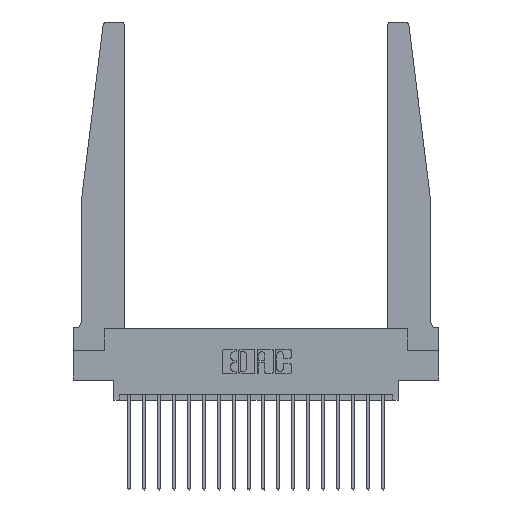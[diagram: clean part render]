
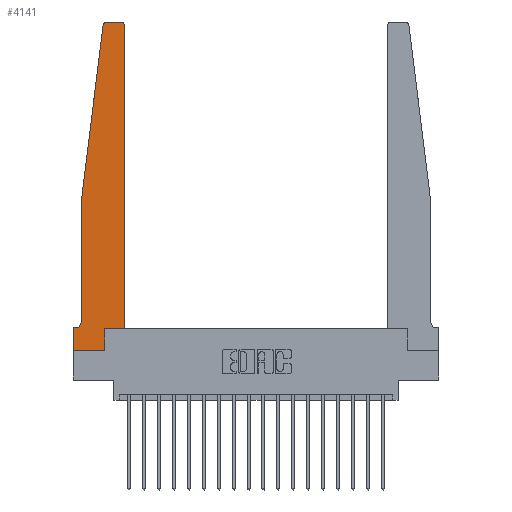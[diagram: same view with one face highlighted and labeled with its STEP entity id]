
A CAD part, top view. The second image highlights one B-rep face of the part: STEP entity #4141.
In plain terms, the highlighted planar face has unit normal (0, 0, 1).
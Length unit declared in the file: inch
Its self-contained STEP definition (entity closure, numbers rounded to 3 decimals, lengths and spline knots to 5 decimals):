
#254 = VERTEX_POINT ( 'NONE', #12240 ) ;
#516 = CARTESIAN_POINT ( 'NONE',  ( 0., 0., 0.37 ) ) ;
#524 = ORIENTED_EDGE ( 'NONE', *, *, #786, .T. ) ;
#786 = EDGE_CURVE ( 'NONE', #16595, #11961, #11822, .T. ) ;
#792 = VERTEX_POINT ( 'NONE', #1582 ) ;
#1427 = EDGE_CURVE ( 'NONE', #10707, #254, #6270, .T. ) ;
#1582 = CARTESIAN_POINT ( 'NONE',  ( 0., 0.1875, 0.37 ) ) ;
#1601 = DIRECTION ( 'NONE',  ( -0.122, -0.992, 0. ) ) ;
#1980 = ORIENTED_EDGE ( 'NONE', *, *, #9373, .T. ) ;
#2039 = CARTESIAN_POINT ( 'NONE',  ( 0., 0., 0.37 ) ) ;
#2236 = ORIENTED_EDGE ( 'NONE', *, *, #12065, .T. ) ;
#2300 = CARTESIAN_POINT ( 'NONE',  ( 0.065, 0.1875, 0.37 ) ) ;
#2331 = EDGE_LOOP ( 'NONE', ( #16674, #18493, #1980, #10214, #2236, #14334, #15579, #4472, #19203, #524, #14915, #15551 ) ) ;
#2355 = FACE_OUTER_BOUND ( 'NONE', #2331, .T. ) ;
#3036 = VERTEX_POINT ( 'NONE', #16102 ) ;
#3189 = VECTOR ( 'NONE', #12989, 39.37008 ) ;
#3217 = LINE ( 'NONE', #516, #19069 ) ;
#3950 = DIRECTION ( 'NONE',  ( -1., 0., 0. ) ) ;
#4141 = ADVANCED_FACE ( 'NONE', ( #2355 ), #6121, .T. ) ;
#4194 = EDGE_CURVE ( 'NONE', #8785, #9283, #17755, .T. ) ;
#4259 = CARTESIAN_POINT ( 'NONE',  ( 0.2605, 0.18, 0.37 ) ) ;
#4472 = ORIENTED_EDGE ( 'NONE', *, *, #1427, .T. ) ;
#4792 = AXIS2_PLACEMENT_3D ( 'NONE', #16905, #7654, #18449 ) ;
#4991 = DIRECTION ( 'NONE',  ( 0., 0., 1. ) ) ;
#5157 = DIRECTION ( 'NONE',  ( 0., 0., -1. ) ) ;
#5566 = CARTESIAN_POINT ( 'NONE',  ( 0.27653, 2.72, 0.37 ) ) ;
#5692 = LINE ( 'NONE', #12302, #8798 ) ;
#6121 = PLANE ( 'NONE',  #4792 ) ;
#6270 = LINE ( 'NONE', #7575, #18107 ) ;
#6414 = DIRECTION ( 'NONE',  ( 0., 1., 0. ) ) ;
#7090 = DIRECTION ( 'NONE',  ( 1., 0., 0. ) ) ;
#7575 = CARTESIAN_POINT ( 'NONE',  ( 0., 0., 0.37 ) ) ;
#7654 = DIRECTION ( 'NONE',  ( 0., 0., 1. ) ) ;
#7961 = CARTESIAN_POINT ( 'NONE',  ( 0.425, 0.18, 0.37 ) ) ;
#8785 = VERTEX_POINT ( 'NONE', #10706 ) ;
#8798 = VECTOR ( 'NONE', #1601, 39.37008 ) ;
#8868 = LINE ( 'NONE', #14680, #17066 ) ;
#9215 = EDGE_CURVE ( 'NONE', #13686, #16363, #15149, .T. ) ;
#9283 = VERTEX_POINT ( 'NONE', #19532 ) ;
#9373 = EDGE_CURVE ( 'NONE', #16363, #8785, #5692, .T. ) ;
#10214 = ORIENTED_EDGE ( 'NONE', *, *, #4194, .T. ) ;
#10706 = CARTESIAN_POINT ( 'NONE',  ( 0.065, 1.25, 0.37 ) ) ;
#10707 = VERTEX_POINT ( 'NONE', #2039 ) ;
#10833 = LINE ( 'NONE', #2300, #3189 ) ;
#11227 = EDGE_CURVE ( 'NONE', #11961, #13892, #16921, .T. ) ;
#11345 = EDGE_CURVE ( 'NONE', #792, #10707, #3217, .T. ) ;
#11695 = CARTESIAN_POINT ( 'NONE',  ( 0.27653, 2.75, 0.37 ) ) ;
#11822 = LINE ( 'NONE', #12413, #14980 ) ;
#11961 = VERTEX_POINT ( 'NONE', #15616 ) ;
#12065 = EDGE_CURVE ( 'NONE', #9283, #3036, #15671, .T. ) ;
#12240 = CARTESIAN_POINT ( 'NONE',  ( 0.2605, 0., 0.37 ) ) ;
#12302 = CARTESIAN_POINT ( 'NONE',  ( 0.065, 1.25, 0.37 ) ) ;
#12355 = AXIS2_PLACEMENT_3D ( 'NONE', #5566, #16315, #7090 ) ;
#12378 = AXIS2_PLACEMENT_3D ( 'NONE', #14344, #5157, #15896 ) ;
#12391 = CARTESIAN_POINT ( 'NONE',  ( 0.065, 1.25, 0.37 ) ) ;
#12413 = CARTESIAN_POINT ( 'NONE',  ( 0.425, 0.18, 0.37 ) ) ;
#12776 = VECTOR ( 'NONE', #6414, 39.37008 ) ;
#12989 = DIRECTION ( 'NONE',  ( -1., 0., 0. ) ) ;
#13686 = VERTEX_POINT ( 'NONE', #11695 ) ;
#13892 = VERTEX_POINT ( 'NONE', #15277 ) ;
#14163 = CARTESIAN_POINT ( 'NONE',  ( 0.395, 2.72, 0.37 ) ) ;
#14173 = VECTOR ( 'NONE', #18573, 39.37008 ) ;
#14334 = ORIENTED_EDGE ( 'NONE', *, *, #18306, .T. ) ;
#14344 = CARTESIAN_POINT ( 'NONE',  ( 0.015, 0.2375, 0.37 ) ) ;
#14680 = CARTESIAN_POINT ( 'NONE',  ( 0.25, 2.75, 0.37 ) ) ;
#14715 = EDGE_CURVE ( 'NONE', #13892, #18227, #16581, .T. ) ;
#14915 = ORIENTED_EDGE ( 'NONE', *, *, #11227, .T. ) ;
#14980 = VECTOR ( 'NONE', #15417, 39.37008 ) ;
#15149 = CIRCLE ( 'NONE', #12355, 0.03 ) ;
#15266 = DIRECTION ( 'NONE',  ( 1., 0., 0. ) ) ;
#15277 = CARTESIAN_POINT ( 'NONE',  ( 0.425, 2.72, 0.37 ) ) ;
#15400 = CARTESIAN_POINT ( 'NONE',  ( 0.2605, 0.18, 0.37 ) ) ;
#15417 = DIRECTION ( 'NONE',  ( 1., 0., 0. ) ) ;
#15542 = DIRECTION ( 'NONE',  ( 0., -1., 0. ) ) ;
#15551 = ORIENTED_EDGE ( 'NONE', *, *, #14715, .T. ) ;
#15555 = AXIS2_PLACEMENT_3D ( 'NONE', #14163, #4991, #15713 ) ;
#15579 = ORIENTED_EDGE ( 'NONE', *, *, #11345, .T. ) ;
#15616 = CARTESIAN_POINT ( 'NONE',  ( 0.425, 0.18, 0.37 ) ) ;
#15671 = CIRCLE ( 'NONE', #12378, 0.05 ) ;
#15713 = DIRECTION ( 'NONE',  ( 1., 0., 0. ) ) ;
#15896 = DIRECTION ( 'NONE',  ( -1., 0., 0. ) ) ;
#15943 = CARTESIAN_POINT ( 'NONE',  ( 0.24675, 2.72367, 0.37 ) ) ;
#16102 = CARTESIAN_POINT ( 'NONE',  ( 0.015, 0.1875, 0.37 ) ) ;
#16315 = DIRECTION ( 'NONE',  ( 0., 0., 1. ) ) ;
#16363 = VERTEX_POINT ( 'NONE', #15943 ) ;
#16581 = CIRCLE ( 'NONE', #15555, 0.03 ) ;
#16595 = VERTEX_POINT ( 'NONE', #4259 ) ;
#16674 = ORIENTED_EDGE ( 'NONE', *, *, #19728, .T. ) ;
#16905 = CARTESIAN_POINT ( 'NONE',  ( 0., 0.1875, 0.37 ) ) ;
#16921 = LINE ( 'NONE', #7961, #12776 ) ;
#17066 = VECTOR ( 'NONE', #3950, 39.37008 ) ;
#17146 = CARTESIAN_POINT ( 'NONE',  ( 0.395, 2.75, 0.37 ) ) ;
#17256 = VECTOR ( 'NONE', #15542, 39.37008 ) ;
#17483 = DIRECTION ( 'NONE',  ( 0., -1., 0. ) ) ;
#17755 = LINE ( 'NONE', #12391, #17256 ) ;
#18107 = VECTOR ( 'NONE', #15266, 39.37008 ) ;
#18227 = VERTEX_POINT ( 'NONE', #17146 ) ;
#18287 = LINE ( 'NONE', #15400, #14173 ) ;
#18306 = EDGE_CURVE ( 'NONE', #3036, #792, #10833, .T. ) ;
#18449 = DIRECTION ( 'NONE',  ( 1., 0., 0. ) ) ;
#18493 = ORIENTED_EDGE ( 'NONE', *, *, #9215, .T. ) ;
#18573 = DIRECTION ( 'NONE',  ( 0., 1., 0. ) ) ;
#19069 = VECTOR ( 'NONE', #17483, 39.37008 ) ;
#19203 = ORIENTED_EDGE ( 'NONE', *, *, #19443, .T. ) ;
#19443 = EDGE_CURVE ( 'NONE', #254, #16595, #18287, .T. ) ;
#19532 = CARTESIAN_POINT ( 'NONE',  ( 0.065, 0.2375, 0.37 ) ) ;
#19728 = EDGE_CURVE ( 'NONE', #18227, #13686, #8868, .T. ) ;
